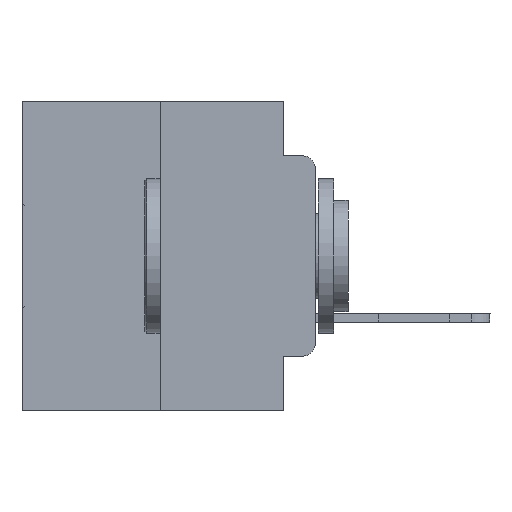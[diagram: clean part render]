
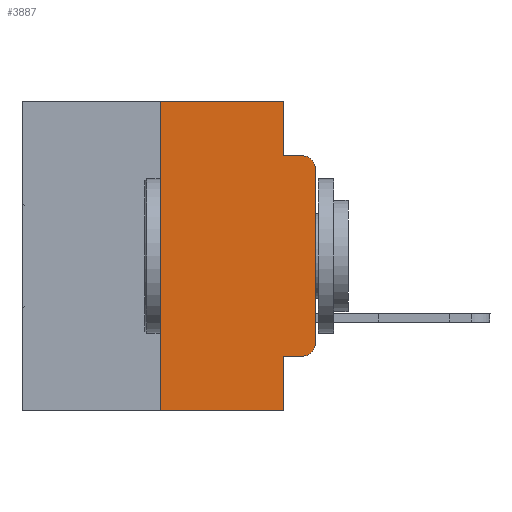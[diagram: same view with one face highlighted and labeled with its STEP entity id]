
A CAD part, left-side view. The second image highlights one B-rep face of the part: STEP entity #3887.
In plain terms, the highlighted planar face has unit normal (-1, 0, 0).
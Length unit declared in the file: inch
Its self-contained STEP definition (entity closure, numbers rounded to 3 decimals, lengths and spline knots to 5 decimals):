
#372 = DIRECTION ( 'NONE',  ( 0., 0., -1. ) ) ;
#658 = CARTESIAN_POINT ( 'NONE',  ( 0., 0., 0. ) ) ;
#760 = EDGE_CURVE ( 'NONE', #23430, #3251, #8915, .T. ) ;
#1888 = CARTESIAN_POINT ( 'NONE',  ( 0., 0.02, -0.3915 ) ) ;
#2467 = EDGE_CURVE ( 'NONE', #17381, #18256, #4166, .T. ) ;
#3251 = VERTEX_POINT ( 'NONE', #12730 ) ;
#3850 = EDGE_LOOP ( 'NONE', ( #16718, #27559, #6732, #4425, #20891, #11004, #14629, #24602, #4123, #26962 ) ) ;
#3887 = ADVANCED_FACE ( 'NONE', ( #9121 ), #23175, .F. ) ;
#4112 = DIRECTION ( 'NONE',  ( 0., 0., 1. ) ) ;
#4123 = ORIENTED_EDGE ( 'NONE', *, *, #12710, .T. ) ;
#4166 = LINE ( 'NONE', #18323, #16142 ) ;
#4413 = CARTESIAN_POINT ( 'NONE',  ( 0., 0.25, 0. ) ) ;
#4425 = ORIENTED_EDGE ( 'NONE', *, *, #8394, .F. ) ;
#4514 = EDGE_CURVE ( 'NONE', #9685, #18243, #15037, .T. ) ;
#4605 = DIRECTION ( 'NONE',  ( 0., 0., -1. ) ) ;
#4674 = VECTOR ( 'NONE', #5121, 39.37008 ) ;
#5111 = VECTOR ( 'NONE', #4605, 39.37008 ) ;
#5121 = DIRECTION ( 'NONE',  ( 0., 0., 1. ) ) ;
#5277 = EDGE_CURVE ( 'NONE', #10719, #27859, #15756, .T. ) ;
#5514 = CARTESIAN_POINT ( 'NONE',  ( 0., 0.051, -0.4115 ) ) ;
#6344 = CARTESIAN_POINT ( 'NONE',  ( 0., 0., -0.1085 ) ) ;
#6489 = DIRECTION ( 'NONE',  ( 0., -1., 0. ) ) ;
#6695 = EDGE_CURVE ( 'NONE', #28358, #27859, #26206, .T. ) ;
#6700 = CARTESIAN_POINT ( 'NONE',  ( 0., 0.02, -0.4115 ) ) ;
#6732 = ORIENTED_EDGE ( 'NONE', *, *, #6695, .F. ) ;
#7303 = CARTESIAN_POINT ( 'NONE',  ( 0., 0.051, 0. ) ) ;
#8394 = EDGE_CURVE ( 'NONE', #18256, #28358, #25707, .T. ) ;
#8770 = DIRECTION ( 'NONE',  ( -1., 0., 0. ) ) ;
#8915 = CIRCLE ( 'NONE', #26176, 0.02 ) ;
#9106 = DIRECTION ( 'NONE',  ( -1., 0., 0. ) ) ;
#9121 = FACE_OUTER_BOUND ( 'NONE', #3850, .T. ) ;
#9685 = VERTEX_POINT ( 'NONE', #24450 ) ;
#9966 = VECTOR ( 'NONE', #4112, 39.37008 ) ;
#10719 = VERTEX_POINT ( 'NONE', #6344 ) ;
#10957 = DIRECTION ( 'NONE',  ( 0., 0., -1. ) ) ;
#11004 = ORIENTED_EDGE ( 'NONE', *, *, #19468, .F. ) ;
#11108 = VECTOR ( 'NONE', #12581, 39.37008 ) ;
#11663 = CARTESIAN_POINT ( 'NONE',  ( 0., 0.051, 0. ) ) ;
#11978 = VERTEX_POINT ( 'NONE', #27456 ) ;
#12581 = DIRECTION ( 'NONE',  ( 0., -1., 0. ) ) ;
#12710 = EDGE_CURVE ( 'NONE', #11978, #23430, #14570, .T. ) ;
#12730 = CARTESIAN_POINT ( 'NONE',  ( 0., 0., -0.3915 ) ) ;
#13760 = AXIS2_PLACEMENT_3D ( 'NONE', #14002, #8770, #28053 ) ;
#14002 = CARTESIAN_POINT ( 'NONE',  ( 0., 0.02, -0.1085 ) ) ;
#14462 = DIRECTION ( 'NONE',  ( 0., -1., 0. ) ) ;
#14570 = LINE ( 'NONE', #5514, #11108 ) ;
#14629 = ORIENTED_EDGE ( 'NONE', *, *, #4514, .T. ) ;
#14805 = EDGE_CURVE ( 'NONE', #11978, #18243, #21462, .T. ) ;
#15037 = LINE ( 'NONE', #21683, #18319 ) ;
#15756 = CIRCLE ( 'NONE', #13760, 0.02 ) ;
#16014 = CARTESIAN_POINT ( 'NONE',  ( 0., 0.02, -0.0885 ) ) ;
#16065 = CARTESIAN_POINT ( 'NONE',  ( 0., 0.051, 0. ) ) ;
#16142 = VECTOR ( 'NONE', #6489, 39.37008 ) ;
#16718 = ORIENTED_EDGE ( 'NONE', *, *, #25059, .T. ) ;
#17381 = VERTEX_POINT ( 'NONE', #27162 ) ;
#18243 = VERTEX_POINT ( 'NONE', #21001 ) ;
#18256 = VERTEX_POINT ( 'NONE', #16065 ) ;
#18319 = VECTOR ( 'NONE', #26476, 39.37008 ) ;
#18323 = CARTESIAN_POINT ( 'NONE',  ( 0., 0.473, 0. ) ) ;
#18521 = DIRECTION ( 'NONE',  ( 1., 0., 0. ) ) ;
#18609 = AXIS2_PLACEMENT_3D ( 'NONE', #23327, #18521, #21298 ) ;
#18679 = VECTOR ( 'NONE', #14462, 39.37008 ) ;
#19468 = EDGE_CURVE ( 'NONE', #9685, #17381, #27838, .T. ) ;
#20891 = ORIENTED_EDGE ( 'NONE', *, *, #2467, .F. ) ;
#21001 = CARTESIAN_POINT ( 'NONE',  ( 0., 0.051, -0.5 ) ) ;
#21298 = DIRECTION ( 'NONE',  ( 0., 0., -1. ) ) ;
#21462 = LINE ( 'NONE', #7303, #22560 ) ;
#21593 = LINE ( 'NONE', #658, #4674 ) ;
#21683 = CARTESIAN_POINT ( 'NONE',  ( 0., 0.473, -0.5 ) ) ;
#21722 = CARTESIAN_POINT ( 'NONE',  ( 0., 0.051, -0.0885 ) ) ;
#22560 = VECTOR ( 'NONE', #372, 39.37008 ) ;
#23175 = PLANE ( 'NONE',  #18609 ) ;
#23327 = CARTESIAN_POINT ( 'NONE',  ( 0., 0.473, 0. ) ) ;
#23430 = VERTEX_POINT ( 'NONE', #6700 ) ;
#23858 = CARTESIAN_POINT ( 'NONE',  ( 0., 0.051, -0.0885 ) ) ;
#24450 = CARTESIAN_POINT ( 'NONE',  ( 0., 0.25, -0.5 ) ) ;
#24602 = ORIENTED_EDGE ( 'NONE', *, *, #14805, .F. ) ;
#25059 = EDGE_CURVE ( 'NONE', #3251, #10719, #21593, .T. ) ;
#25707 = LINE ( 'NONE', #11663, #5111 ) ;
#26176 = AXIS2_PLACEMENT_3D ( 'NONE', #1888, #9106, #10957 ) ;
#26206 = LINE ( 'NONE', #21722, #18679 ) ;
#26476 = DIRECTION ( 'NONE',  ( 0., -1., 0. ) ) ;
#26962 = ORIENTED_EDGE ( 'NONE', *, *, #760, .T. ) ;
#27162 = CARTESIAN_POINT ( 'NONE',  ( 0., 0.25, 0. ) ) ;
#27456 = CARTESIAN_POINT ( 'NONE',  ( 0., 0.051, -0.4115 ) ) ;
#27559 = ORIENTED_EDGE ( 'NONE', *, *, #5277, .T. ) ;
#27838 = LINE ( 'NONE', #4413, #9966 ) ;
#27859 = VERTEX_POINT ( 'NONE', #16014 ) ;
#28053 = DIRECTION ( 'NONE',  ( 0., 0., -1. ) ) ;
#28358 = VERTEX_POINT ( 'NONE', #23858 ) ;
